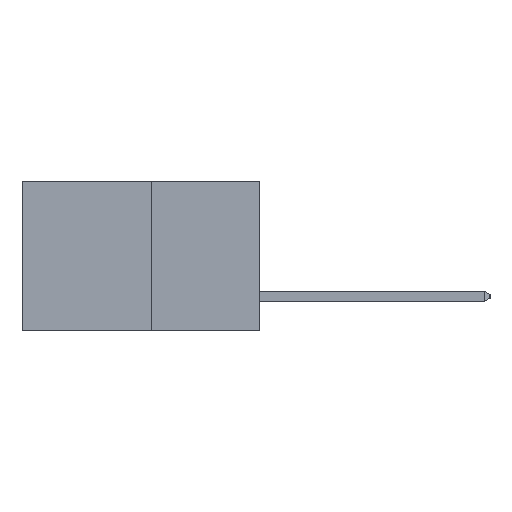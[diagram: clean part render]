
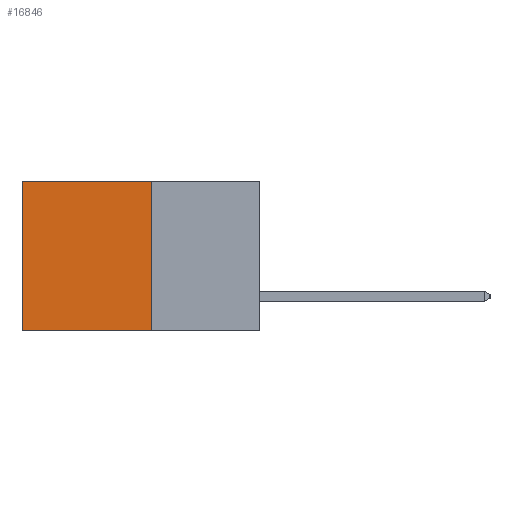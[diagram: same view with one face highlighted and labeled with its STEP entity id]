
A CAD part, left-side view. The second image highlights one B-rep face of the part: STEP entity #16846.
In plain terms, the highlighted planar face has unit normal (-1, 0, 0).
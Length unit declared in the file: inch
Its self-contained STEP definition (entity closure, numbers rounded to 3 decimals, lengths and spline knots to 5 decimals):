
#948 = EDGE_CURVE ( 'NONE', #14034, #24027, #23942, .T. ) ;
#1226 = CARTESIAN_POINT ( 'NONE',  ( 0.277, 0.59, -0.37 ) ) ;
#2271 = CARTESIAN_POINT ( 'NONE',  ( 0.277, 0.27, -0.37 ) ) ;
#2302 = DIRECTION ( 'NONE',  ( 1., 0., 0. ) ) ;
#2797 = CARTESIAN_POINT ( 'NONE',  ( 0.277, 0.27, -0.37 ) ) ;
#3314 = DIRECTION ( 'NONE',  ( 0., 0., -1. ) ) ;
#3716 = LINE ( 'NONE', #23689, #20184 ) ;
#6084 = LINE ( 'NONE', #12180, #16405 ) ;
#6997 = EDGE_LOOP ( 'NONE', ( #17348, #9742, #12939, #26166 ) ) ;
#8207 = VECTOR ( 'NONE', #3314, 39.37008 ) ;
#9742 = ORIENTED_EDGE ( 'NONE', *, *, #20644, .F. ) ;
#9975 = DIRECTION ( 'NONE',  ( 0., 0., -1. ) ) ;
#10747 = AXIS2_PLACEMENT_3D ( 'NONE', #18728, #2302, #16742 ) ;
#12180 = CARTESIAN_POINT ( 'NONE',  ( 0.277, 0.27, -0.37 ) ) ;
#12939 = ORIENTED_EDGE ( 'NONE', *, *, #948, .F. ) ;
#13248 = VERTEX_POINT ( 'NONE', #18231 ) ;
#14034 = VERTEX_POINT ( 'NONE', #20227 ) ;
#14266 = DIRECTION ( 'NONE',  ( 0., 1., 0. ) ) ;
#14687 = PLANE ( 'NONE',  #10747 ) ;
#15273 = FACE_OUTER_BOUND ( 'NONE', #6997, .T. ) ;
#16405 = VECTOR ( 'NONE', #14266, 39.37008 ) ;
#16742 = DIRECTION ( 'NONE',  ( 0., 0., -1. ) ) ;
#16846 = ADVANCED_FACE ( 'NONE', ( #15273 ), #14687, .F. ) ;
#17348 = ORIENTED_EDGE ( 'NONE', *, *, #22846, .T. ) ;
#18231 = CARTESIAN_POINT ( 'NONE',  ( 0.277, 0.59, -0.37 ) ) ;
#18728 = CARTESIAN_POINT ( 'NONE',  ( 0.277, 0.27, -0.37 ) ) ;
#19110 = VECTOR ( 'NONE', #9975, 39.37008 ) ;
#19187 = LINE ( 'NONE', #1226, #8207 ) ;
#20184 = VECTOR ( 'NONE', #23601, 39.37008 ) ;
#20227 = CARTESIAN_POINT ( 'NONE',  ( 0.277, 0.27, 0. ) ) ;
#20644 = EDGE_CURVE ( 'NONE', #24027, #13248, #6084, .T. ) ;
#21210 = VERTEX_POINT ( 'NONE', #26283 ) ;
#22846 = EDGE_CURVE ( 'NONE', #21210, #13248, #19187, .T. ) ;
#23601 = DIRECTION ( 'NONE',  ( 0., 1., 0. ) ) ;
#23689 = CARTESIAN_POINT ( 'NONE',  ( 0.277, 0.27, 0. ) ) ;
#23942 = LINE ( 'NONE', #2271, #19110 ) ;
#24027 = VERTEX_POINT ( 'NONE', #2797 ) ;
#25756 = EDGE_CURVE ( 'NONE', #14034, #21210, #3716, .T. ) ;
#26166 = ORIENTED_EDGE ( 'NONE', *, *, #25756, .T. ) ;
#26283 = CARTESIAN_POINT ( 'NONE',  ( 0.277, 0.59, 0. ) ) ;
